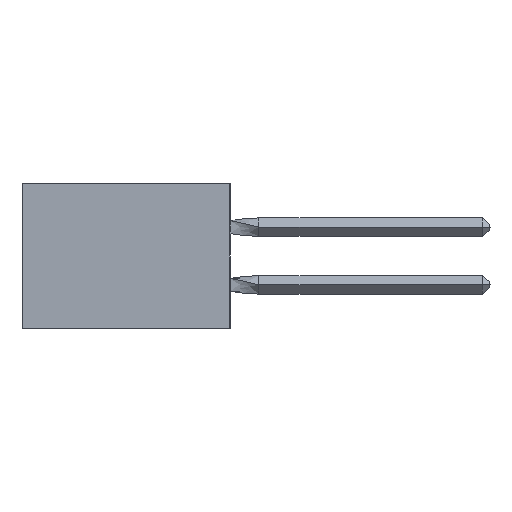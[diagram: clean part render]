
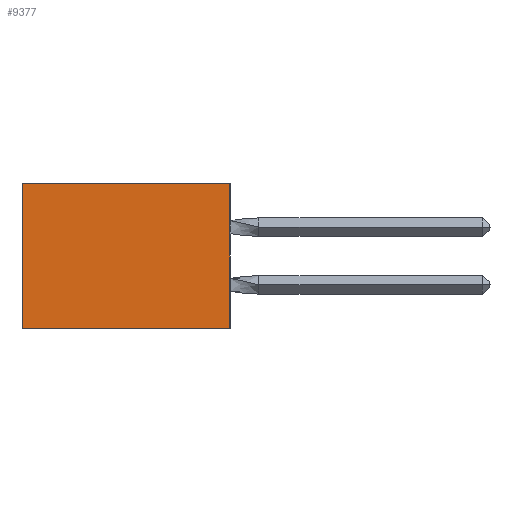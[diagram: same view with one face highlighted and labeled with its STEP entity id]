
A CAD part, left-side view. The second image highlights one B-rep face of the part: STEP entity #9377.
In plain terms, the highlighted planar face has unit normal (-1, 0, 0).
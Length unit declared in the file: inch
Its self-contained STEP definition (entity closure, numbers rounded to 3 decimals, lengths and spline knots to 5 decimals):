
#715 = LINE ( 'NONE', #34948, #18002 ) ;
#4510 = DIRECTION ( 'NONE',  ( 0., 0., -1. ) ) ;
#4556 = VECTOR ( 'NONE', #27984, 39.37008 ) ;
#7151 = LINE ( 'NONE', #23131, #20758 ) ;
#7885 = AXIS2_PLACEMENT_3D ( 'NONE', #17122, #20482, #4510 ) ;
#9377 = ADVANCED_FACE ( 'NONE', ( #29112 ), #13590, .F. ) ;
#9795 = CARTESIAN_POINT ( 'NONE',  ( 0.305, 0.72, 0. ) ) ;
#11509 = ORIENTED_EDGE ( 'NONE', *, *, #36001, .F. ) ;
#12494 = VERTEX_POINT ( 'NONE', #29621 ) ;
#13306 = VERTEX_POINT ( 'NONE', #9795 ) ;
#13590 = PLANE ( 'NONE',  #7885 ) ;
#14709 = CARTESIAN_POINT ( 'NONE',  ( 0.305, 0., -0.5 ) ) ;
#15174 = DIRECTION ( 'NONE',  ( 0., 1., 0. ) ) ;
#16902 = LINE ( 'NONE', #14709, #23187 ) ;
#17052 = EDGE_CURVE ( 'NONE', #27265, #21813, #16902, .T. ) ;
#17122 = CARTESIAN_POINT ( 'NONE',  ( 0.305, 0., -0.5 ) ) ;
#17448 = CARTESIAN_POINT ( 'NONE',  ( 0.305, 0., 0. ) ) ;
#18002 = VECTOR ( 'NONE', #15174, 39.37008 ) ;
#19517 = EDGE_CURVE ( 'NONE', #13306, #12494, #7151, .T. ) ;
#20482 = DIRECTION ( 'NONE',  ( 1., 0., 0. ) ) ;
#20758 = VECTOR ( 'NONE', #42472, 39.37008 ) ;
#21704 = CARTESIAN_POINT ( 'NONE',  ( 0.305, 0., -0.5 ) ) ;
#21813 = VERTEX_POINT ( 'NONE', #31644 ) ;
#23131 = CARTESIAN_POINT ( 'NONE',  ( 0.305, 0.72, -0.5 ) ) ;
#23187 = VECTOR ( 'NONE', #38400, 39.37008 ) ;
#26551 = ORIENTED_EDGE ( 'NONE', *, *, #17052, .F. ) ;
#26793 = EDGE_LOOP ( 'NONE', ( #33823, #11509, #26551, #37747 ) ) ;
#27265 = VERTEX_POINT ( 'NONE', #17448 ) ;
#27984 = DIRECTION ( 'NONE',  ( 0., 1., 0. ) ) ;
#29112 = FACE_OUTER_BOUND ( 'NONE', #26793, .T. ) ;
#29621 = CARTESIAN_POINT ( 'NONE',  ( 0.305, 0.72, -0.5 ) ) ;
#31644 = CARTESIAN_POINT ( 'NONE',  ( 0.305, 0., -0.5 ) ) ;
#32527 = EDGE_CURVE ( 'NONE', #27265, #13306, #715, .T. ) ;
#33823 = ORIENTED_EDGE ( 'NONE', *, *, #19517, .T. ) ;
#34948 = CARTESIAN_POINT ( 'NONE',  ( 0.305, 0., 0. ) ) ;
#36001 = EDGE_CURVE ( 'NONE', #21813, #12494, #39155, .T. ) ;
#37747 = ORIENTED_EDGE ( 'NONE', *, *, #32527, .T. ) ;
#38400 = DIRECTION ( 'NONE',  ( 0., 0., -1. ) ) ;
#39155 = LINE ( 'NONE', #21704, #4556 ) ;
#42472 = DIRECTION ( 'NONE',  ( 0., 0., -1. ) ) ;
